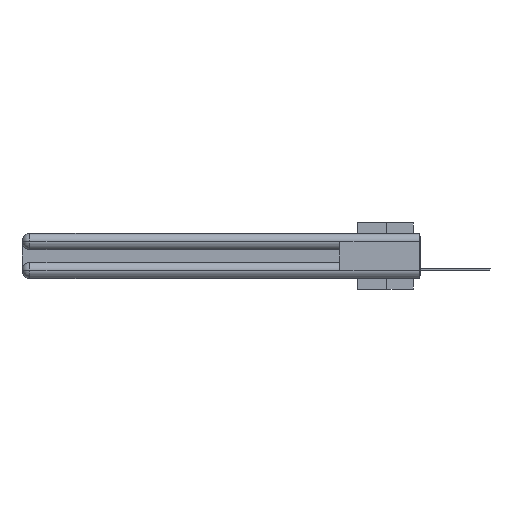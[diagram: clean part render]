
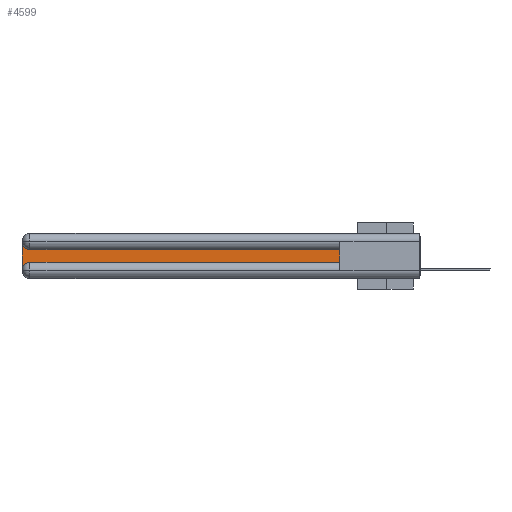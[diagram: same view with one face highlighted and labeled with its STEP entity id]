
A CAD part, left-side view. The second image highlights one B-rep face of the part: STEP entity #4599.
In plain terms, the highlighted planar face has unit normal (-1, 0, 0).
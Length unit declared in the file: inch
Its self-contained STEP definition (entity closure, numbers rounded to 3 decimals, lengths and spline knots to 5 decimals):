
#298 = CARTESIAN_POINT ( 'NONE',  ( 0.075, 3., -0.0625 ) ) ;
#580 = DIRECTION ( 'NONE',  ( 0., -1., 0. ) ) ;
#1714 = PLANE ( 'NONE',  #10474 ) ;
#1785 = CIRCLE ( 'NONE', #19647, 0.06 ) ;
#2740 = EDGE_CURVE ( 'NONE', #7579, #4940, #8016, .T. ) ;
#3414 = LINE ( 'NONE', #13923, #20200 ) ;
#3565 = DIRECTION ( 'NONE',  ( 0., 0., -1. ) ) ;
#4204 = DIRECTION ( 'NONE',  ( 0., 0., -1. ) ) ;
#4599 = ADVANCED_FACE ( 'NONE', ( #11697 ), #1714, .F. ) ;
#4940 = VERTEX_POINT ( 'NONE', #32078 ) ;
#5211 = CIRCLE ( 'NONE', #32290, 0.06 ) ;
#5269 = DIRECTION ( 'NONE',  ( 0., 0., -1. ) ) ;
#5697 = CARTESIAN_POINT ( 'NONE',  ( 0.075, 0.6, -0.1225 ) ) ;
#7579 = VERTEX_POINT ( 'NONE', #20221 ) ;
#7718 = ORIENTED_EDGE ( 'NONE', *, *, #29672, .T. ) ;
#7755 = EDGE_CURVE ( 'NONE', #10913, #22387, #21711, .T. ) ;
#8016 = LINE ( 'NONE', #18533, #29892 ) ;
#8476 = CARTESIAN_POINT ( 'NONE',  ( 0.075, 3., -0.2175 ) ) ;
#8811 = DIRECTION ( 'NONE',  ( 0., 0., -1. ) ) ;
#9484 = VECTOR ( 'NONE', #3565, 39.37008 ) ;
#10474 = AXIS2_PLACEMENT_3D ( 'NONE', #22412, #32045, #8811 ) ;
#10913 = VERTEX_POINT ( 'NONE', #298 ) ;
#11697 = FACE_OUTER_BOUND ( 'NONE', #17220, .T. ) ;
#12287 = CARTESIAN_POINT ( 'NONE',  ( 0.075, 3., -0.2775 ) ) ;
#12669 = ORIENTED_EDGE ( 'NONE', *, *, #14405, .T. ) ;
#13923 = CARTESIAN_POINT ( 'NONE',  ( 0.075, 0.6, -0.1225 ) ) ;
#14405 = EDGE_CURVE ( 'NONE', #27283, #10913, #1785, .T. ) ;
#14424 = ORIENTED_EDGE ( 'NONE', *, *, #31568, .T. ) ;
#15289 = EDGE_CURVE ( 'NONE', #25279, #27283, #3414, .T. ) ;
#17220 = EDGE_LOOP ( 'NONE', ( #18941, #12669, #32915, #14424, #31523, #7718 ) ) ;
#17860 = DIRECTION ( 'NONE',  ( 0., 0., 1. ) ) ;
#18533 = CARTESIAN_POINT ( 'NONE',  ( 0.075, 0.6, -0.2175 ) ) ;
#18941 = ORIENTED_EDGE ( 'NONE', *, *, #15289, .T. ) ;
#19647 = AXIS2_PLACEMENT_3D ( 'NONE', #27123, #32696, #4204 ) ;
#20200 = VECTOR ( 'NONE', #24135, 39.37008 ) ;
#20221 = CARTESIAN_POINT ( 'NONE',  ( 0.075, 2.94, -0.2175 ) ) ;
#21711 = LINE ( 'NONE', #8476, #9484 ) ;
#22387 = VERTEX_POINT ( 'NONE', #12287 ) ;
#22412 = CARTESIAN_POINT ( 'NONE',  ( 0.075, 3., -0.1225 ) ) ;
#24135 = DIRECTION ( 'NONE',  ( 0., 1., 0. ) ) ;
#24871 = CARTESIAN_POINT ( 'NONE',  ( 0.075, 0.6, -0.2175 ) ) ;
#25279 = VERTEX_POINT ( 'NONE', #5697 ) ;
#27123 = CARTESIAN_POINT ( 'NONE',  ( 0.075, 2.94, -0.0625 ) ) ;
#27283 = VERTEX_POINT ( 'NONE', #27543 ) ;
#27543 = CARTESIAN_POINT ( 'NONE',  ( 0.075, 2.94, -0.1225 ) ) ;
#29017 = CARTESIAN_POINT ( 'NONE',  ( 0.075, 2.94, -0.2775 ) ) ;
#29672 = EDGE_CURVE ( 'NONE', #4940, #25279, #30260, .T. ) ;
#29892 = VECTOR ( 'NONE', #580, 39.37008 ) ;
#30260 = LINE ( 'NONE', #24871, #33286 ) ;
#30893 = DIRECTION ( 'NONE',  ( 1., 0., 0. ) ) ;
#31523 = ORIENTED_EDGE ( 'NONE', *, *, #2740, .T. ) ;
#31568 = EDGE_CURVE ( 'NONE', #22387, #7579, #5211, .T. ) ;
#32045 = DIRECTION ( 'NONE',  ( 1., 0., 0. ) ) ;
#32078 = CARTESIAN_POINT ( 'NONE',  ( 0.075, 0.6, -0.2175 ) ) ;
#32290 = AXIS2_PLACEMENT_3D ( 'NONE', #29017, #30893, #5269 ) ;
#32696 = DIRECTION ( 'NONE',  ( 1., 0., 0. ) ) ;
#32915 = ORIENTED_EDGE ( 'NONE', *, *, #7755, .T. ) ;
#33286 = VECTOR ( 'NONE', #17860, 39.37008 ) ;
